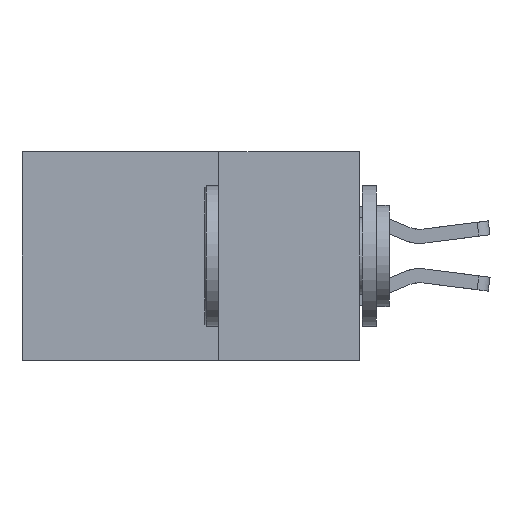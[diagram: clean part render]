
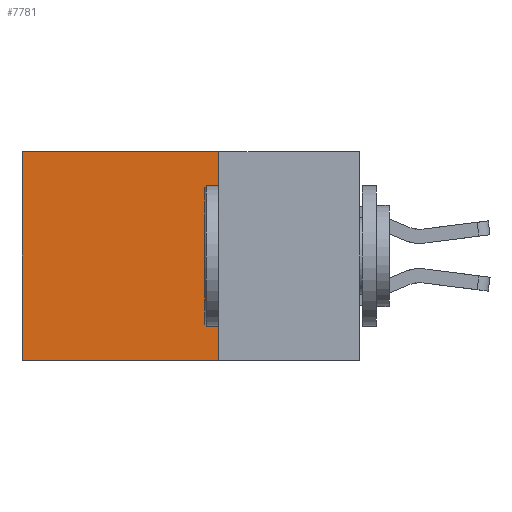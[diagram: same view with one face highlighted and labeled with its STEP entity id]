
A CAD part, left-side view. The second image highlights one B-rep face of the part: STEP entity #7781.
In plain terms, the highlighted planar face has unit normal (-1, 0, 0).
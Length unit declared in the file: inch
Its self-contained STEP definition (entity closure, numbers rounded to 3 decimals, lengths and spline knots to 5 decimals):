
#164 = VERTEX_POINT ( 'NONE', #6887 ) ;
#586 = CARTESIAN_POINT ( 'NONE',  ( 0.2875, 0.6, 0. ) ) ;
#821 = FACE_OUTER_BOUND ( 'NONE', #14449, .T. ) ;
#1591 = VECTOR ( 'NONE', #9426, 39.37008 ) ;
#1976 = CARTESIAN_POINT ( 'NONE',  ( 0.2875, 0.25, 0. ) ) ;
#2514 = ORIENTED_EDGE ( 'NONE', *, *, #4234, .F. ) ;
#2794 = VERTEX_POINT ( 'NONE', #3891 ) ;
#3289 = ORIENTED_EDGE ( 'NONE', *, *, #10231, .T. ) ;
#3671 = EDGE_CURVE ( 'NONE', #2794, #164, #12980, .T. ) ;
#3891 = CARTESIAN_POINT ( 'NONE',  ( 0.2875, 0.6, 0. ) ) ;
#3939 = CARTESIAN_POINT ( 'NONE',  ( 0.2875, 0.25, 0. ) ) ;
#4234 = EDGE_CURVE ( 'NONE', #11796, #5216, #7754, .T. ) ;
#4912 = LINE ( 'NONE', #7198, #1591 ) ;
#5216 = VERTEX_POINT ( 'NONE', #9850 ) ;
#5248 = AXIS2_PLACEMENT_3D ( 'NONE', #14388, #9011, #12342 ) ;
#6467 = CARTESIAN_POINT ( 'NONE',  ( 0.2875, 0.25, 0. ) ) ;
#6586 = EDGE_CURVE ( 'NONE', #5216, #164, #4912, .T. ) ;
#6887 = CARTESIAN_POINT ( 'NONE',  ( 0.2875, 0.6, -0.37 ) ) ;
#7198 = CARTESIAN_POINT ( 'NONE',  ( 0.2875, 0.25, -0.37 ) ) ;
#7301 = VECTOR ( 'NONE', #10759, 39.37008 ) ;
#7636 = LINE ( 'NONE', #1976, #7301 ) ;
#7754 = LINE ( 'NONE', #3939, #8789 ) ;
#7781 = ADVANCED_FACE ( 'NONE', ( #821 ), #7791, .F. ) ;
#7791 = PLANE ( 'NONE',  #5248 ) ;
#8073 = ORIENTED_EDGE ( 'NONE', *, *, #3671, .T. ) ;
#8789 = VECTOR ( 'NONE', #10518, 39.37008 ) ;
#9011 = DIRECTION ( 'NONE',  ( 1., 0., 0. ) ) ;
#9426 = DIRECTION ( 'NONE',  ( 0., 1., 0. ) ) ;
#9850 = CARTESIAN_POINT ( 'NONE',  ( 0.2875, 0.25, -0.37 ) ) ;
#10231 = EDGE_CURVE ( 'NONE', #11796, #2794, #7636, .T. ) ;
#10518 = DIRECTION ( 'NONE',  ( 0., 0., -1. ) ) ;
#10720 = DIRECTION ( 'NONE',  ( 0., 0., -1. ) ) ;
#10759 = DIRECTION ( 'NONE',  ( 0., 1., 0. ) ) ;
#11796 = VERTEX_POINT ( 'NONE', #6467 ) ;
#12266 = VECTOR ( 'NONE', #10720, 39.37008 ) ;
#12279 = ORIENTED_EDGE ( 'NONE', *, *, #6586, .F. ) ;
#12342 = DIRECTION ( 'NONE',  ( 0., 0., -1. ) ) ;
#12980 = LINE ( 'NONE', #586, #12266 ) ;
#14388 = CARTESIAN_POINT ( 'NONE',  ( 0.2875, 0.25, 0. ) ) ;
#14449 = EDGE_LOOP ( 'NONE', ( #8073, #12279, #2514, #3289 ) ) ;
